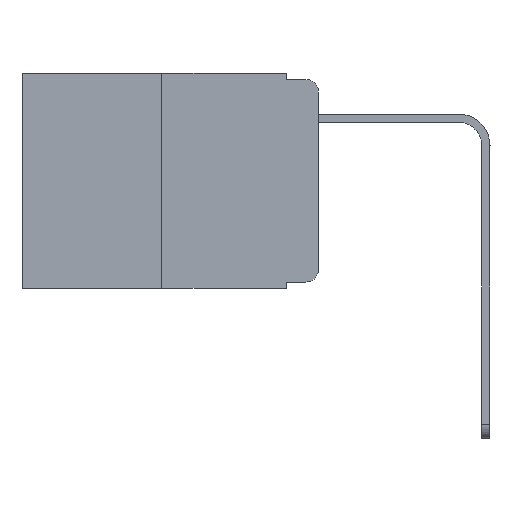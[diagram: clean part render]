
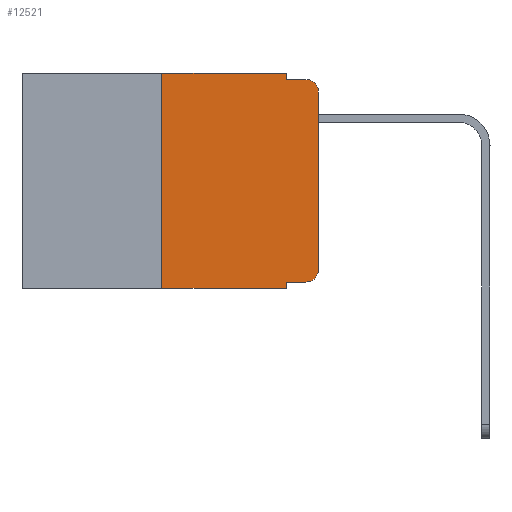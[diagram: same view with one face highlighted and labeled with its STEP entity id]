
A CAD part, left-side view. The second image highlights one B-rep face of the part: STEP entity #12521.
In plain terms, the highlighted planar face has unit normal (-1, 0, 0).
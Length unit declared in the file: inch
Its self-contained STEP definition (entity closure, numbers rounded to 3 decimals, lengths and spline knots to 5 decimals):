
#183 = DIRECTION ( 'NONE',  ( 0., -1., 0. ) ) ;
#320 = LINE ( 'NONE', #12170, #15744 ) ;
#551 = CIRCLE ( 'NONE', #3144, 0.02 ) ;
#718 = CARTESIAN_POINT ( 'NONE',  ( 0., 0.25, 0. ) ) ;
#975 = LINE ( 'NONE', #6324, #12569 ) ;
#1011 = LINE ( 'NONE', #718, #12985 ) ;
#1350 = EDGE_CURVE ( 'NONE', #4892, #3927, #975, .T. ) ;
#1471 = EDGE_CURVE ( 'NONE', #13585, #3927, #10426, .T. ) ;
#1728 = VECTOR ( 'NONE', #14836, 39.37008 ) ;
#1876 = DIRECTION ( 'NONE',  ( 0., 0., 1. ) ) ;
#1994 = ORIENTED_EDGE ( 'NONE', *, *, #3084, .F. ) ;
#2024 = ORIENTED_EDGE ( 'NONE', *, *, #10524, .F. ) ;
#2043 = CARTESIAN_POINT ( 'NONE',  ( 0., 0.051, 0. ) ) ;
#2653 = DIRECTION ( 'NONE',  ( 0., 0., 1. ) ) ;
#3084 = EDGE_CURVE ( 'NONE', #13288, #12837, #8485, .T. ) ;
#3144 = AXIS2_PLACEMENT_3D ( 'NONE', #9659, #3348, #10774 ) ;
#3348 = DIRECTION ( 'NONE',  ( -1., 0., 0. ) ) ;
#3733 = LINE ( 'NONE', #3889, #9916 ) ;
#3889 = CARTESIAN_POINT ( 'NONE',  ( 0., 0.051, -0.333 ) ) ;
#3927 = VERTEX_POINT ( 'NONE', #14201 ) ;
#4088 = VERTEX_POINT ( 'NONE', #4723 ) ;
#4495 = EDGE_CURVE ( 'NONE', #8399, #4088, #320, .T. ) ;
#4627 = DIRECTION ( 'NONE',  ( -1., 0., 0. ) ) ;
#4707 = ORIENTED_EDGE ( 'NONE', *, *, #8728, .T. ) ;
#4723 = CARTESIAN_POINT ( 'NONE',  ( 0., 0.02, -0.01 ) ) ;
#4726 = PLANE ( 'NONE',  #5223 ) ;
#4772 = VECTOR ( 'NONE', #13305, 39.37008 ) ;
#4892 = VERTEX_POINT ( 'NONE', #15383 ) ;
#5181 = CARTESIAN_POINT ( 'NONE',  ( 0., 0.473, 0. ) ) ;
#5223 = AXIS2_PLACEMENT_3D ( 'NONE', #12300, #12247, #7268 ) ;
#5365 = LINE ( 'NONE', #10838, #4772 ) ;
#5570 = ORIENTED_EDGE ( 'NONE', *, *, #1350, .T. ) ;
#5655 = CARTESIAN_POINT ( 'NONE',  ( 0., 0.02, -0.03 ) ) ;
#5866 = DIRECTION ( 'NONE',  ( 0., 0., -1. ) ) ;
#5887 = ORIENTED_EDGE ( 'NONE', *, *, #4495, .F. ) ;
#6127 = CARTESIAN_POINT ( 'NONE',  ( 0., 0.051, 0. ) ) ;
#6272 = VERTEX_POINT ( 'NONE', #10816 ) ;
#6324 = CARTESIAN_POINT ( 'NONE',  ( 0., 0.473, -0.343 ) ) ;
#6599 = EDGE_LOOP ( 'NONE', ( #4707, #11621, #5887, #15769, #1994, #2024, #5570, #14254, #12997, #7453 ) ) ;
#7268 = DIRECTION ( 'NONE',  ( 0., 0., -1. ) ) ;
#7453 = ORIENTED_EDGE ( 'NONE', *, *, #15665, .T. ) ;
#7867 = CARTESIAN_POINT ( 'NONE',  ( 0., 0., -0.03 ) ) ;
#8338 = EDGE_CURVE ( 'NONE', #12837, #8399, #5365, .T. ) ;
#8356 = CARTESIAN_POINT ( 'NONE',  ( 0., 0.051, -0.01 ) ) ;
#8399 = VERTEX_POINT ( 'NONE', #8356 ) ;
#8485 = LINE ( 'NONE', #5181, #1728 ) ;
#8490 = CARTESIAN_POINT ( 'NONE',  ( 0., 0.051, -0.333 ) ) ;
#8728 = EDGE_CURVE ( 'NONE', #15455, #11087, #12464, .T. ) ;
#9095 = FACE_OUTER_BOUND ( 'NONE', #6599, .T. ) ;
#9210 = VECTOR ( 'NONE', #2653, 39.37008 ) ;
#9659 = CARTESIAN_POINT ( 'NONE',  ( 0., 0.02, -0.313 ) ) ;
#9916 = VECTOR ( 'NONE', #11172, 39.37008 ) ;
#10426 = LINE ( 'NONE', #2043, #12937 ) ;
#10524 = EDGE_CURVE ( 'NONE', #4892, #13288, #1011, .T. ) ;
#10644 = DIRECTION ( 'NONE',  ( 0., 0., -1. ) ) ;
#10774 = DIRECTION ( 'NONE',  ( 0., 0., -1. ) ) ;
#10808 = CIRCLE ( 'NONE', #11912, 0.02 ) ;
#10816 = CARTESIAN_POINT ( 'NONE',  ( 0., 0.02, -0.333 ) ) ;
#10838 = CARTESIAN_POINT ( 'NONE',  ( 0., 0.051, 0. ) ) ;
#11087 = VERTEX_POINT ( 'NONE', #7867 ) ;
#11172 = DIRECTION ( 'NONE',  ( 0., -1., 0. ) ) ;
#11621 = ORIENTED_EDGE ( 'NONE', *, *, #11798, .T. ) ;
#11798 = EDGE_CURVE ( 'NONE', #11087, #4088, #10808, .T. ) ;
#11912 = AXIS2_PLACEMENT_3D ( 'NONE', #5655, #4627, #5866 ) ;
#12170 = CARTESIAN_POINT ( 'NONE',  ( 0., 0.051, -0.01 ) ) ;
#12226 = DIRECTION ( 'NONE',  ( 0., -1., 0. ) ) ;
#12247 = DIRECTION ( 'NONE',  ( 1., 0., 0. ) ) ;
#12300 = CARTESIAN_POINT ( 'NONE',  ( 0., 0.473, 0. ) ) ;
#12464 = LINE ( 'NONE', #15087, #9210 ) ;
#12521 = ADVANCED_FACE ( 'NONE', ( #9095 ), #4726, .F. ) ;
#12569 = VECTOR ( 'NONE', #183, 39.37008 ) ;
#12716 = EDGE_CURVE ( 'NONE', #13585, #6272, #3733, .T. ) ;
#12837 = VERTEX_POINT ( 'NONE', #6127 ) ;
#12937 = VECTOR ( 'NONE', #10644, 39.37008 ) ;
#12985 = VECTOR ( 'NONE', #1876, 39.37008 ) ;
#12997 = ORIENTED_EDGE ( 'NONE', *, *, #12716, .T. ) ;
#13288 = VERTEX_POINT ( 'NONE', #15355 ) ;
#13305 = DIRECTION ( 'NONE',  ( 0., 0., -1. ) ) ;
#13585 = VERTEX_POINT ( 'NONE', #8490 ) ;
#14201 = CARTESIAN_POINT ( 'NONE',  ( 0., 0.051, -0.343 ) ) ;
#14254 = ORIENTED_EDGE ( 'NONE', *, *, #1471, .F. ) ;
#14789 = CARTESIAN_POINT ( 'NONE',  ( 0., 0., -0.313 ) ) ;
#14836 = DIRECTION ( 'NONE',  ( 0., -1., 0. ) ) ;
#15087 = CARTESIAN_POINT ( 'NONE',  ( 0., 0., 0. ) ) ;
#15355 = CARTESIAN_POINT ( 'NONE',  ( 0., 0.25, 0. ) ) ;
#15383 = CARTESIAN_POINT ( 'NONE',  ( 0., 0.25, -0.343 ) ) ;
#15455 = VERTEX_POINT ( 'NONE', #14789 ) ;
#15665 = EDGE_CURVE ( 'NONE', #6272, #15455, #551, .T. ) ;
#15744 = VECTOR ( 'NONE', #12226, 39.37008 ) ;
#15769 = ORIENTED_EDGE ( 'NONE', *, *, #8338, .F. ) ;
